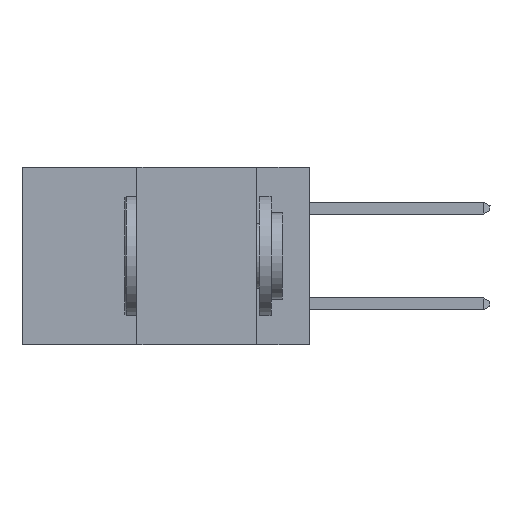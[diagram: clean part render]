
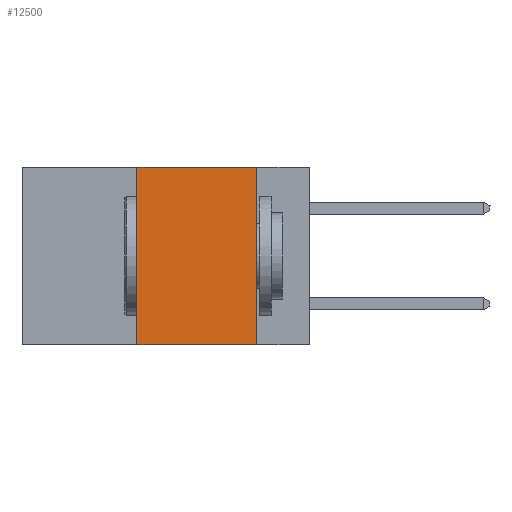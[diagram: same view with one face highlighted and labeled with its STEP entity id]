
A CAD part, left-side view. The second image highlights one B-rep face of the part: STEP entity #12500.
In plain terms, the highlighted planar face has unit normal (-1, 0, 0).
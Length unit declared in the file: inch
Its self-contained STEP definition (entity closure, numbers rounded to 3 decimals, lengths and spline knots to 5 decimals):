
#22 = ORIENTED_EDGE ( 'NONE', *, *, #7633, .F. ) ;
#242 = ORIENTED_EDGE ( 'NONE', *, *, #12107, .F. ) ;
#319 = ORIENTED_EDGE ( 'NONE', *, *, #15485, .F. ) ;
#1530 = ORIENTED_EDGE ( 'NONE', *, *, #19154, .T. ) ;
#2858 = VERTEX_POINT ( 'NONE', #14067 ) ;
#2990 = CARTESIAN_POINT ( 'NONE',  ( 0., 0.11, 0. ) ) ;
#3079 = VECTOR ( 'NONE', #8066, 39.37008 ) ;
#3579 = LINE ( 'NONE', #18610, #3079 ) ;
#5143 = VERTEX_POINT ( 'NONE', #9346 ) ;
#5203 = CARTESIAN_POINT ( 'NONE',  ( 0., 0.11, -0.37 ) ) ;
#5963 = AXIS2_PLACEMENT_3D ( 'NONE', #9404, #16978, #7877 ) ;
#6797 = CARTESIAN_POINT ( 'NONE',  ( 0., 0.6, 0. ) ) ;
#7076 = VERTEX_POINT ( 'NONE', #5203 ) ;
#7633 = EDGE_CURVE ( 'NONE', #13668, #7076, #3579, .T. ) ;
#7877 = DIRECTION ( 'NONE',  ( 0., 0., -1. ) ) ;
#8066 = DIRECTION ( 'NONE',  ( 0., 0., -1. ) ) ;
#9346 = CARTESIAN_POINT ( 'NONE',  ( 0., 0.36, -0.37 ) ) ;
#9404 = CARTESIAN_POINT ( 'NONE',  ( 0., 0.6, 0. ) ) ;
#9689 = CARTESIAN_POINT ( 'NONE',  ( 0., 0.36, 0. ) ) ;
#10066 = LINE ( 'NONE', #9689, #17588 ) ;
#10252 = EDGE_LOOP ( 'NONE', ( #22, #242, #319, #1530 ) ) ;
#10405 = CARTESIAN_POINT ( 'NONE',  ( 0., 0.6, -0.37 ) ) ;
#11948 = FACE_OUTER_BOUND ( 'NONE', #10252, .T. ) ;
#11968 = LINE ( 'NONE', #6797, #15439 ) ;
#12107 = EDGE_CURVE ( 'NONE', #2858, #13668, #11968, .T. ) ;
#12474 = PLANE ( 'NONE',  #5963 ) ;
#12500 = ADVANCED_FACE ( 'NONE', ( #11948 ), #12474, .F. ) ;
#13668 = VERTEX_POINT ( 'NONE', #2990 ) ;
#14067 = CARTESIAN_POINT ( 'NONE',  ( 0., 0.36, 0. ) ) ;
#15439 = VECTOR ( 'NONE', #18910, 39.37008 ) ;
#15485 = EDGE_CURVE ( 'NONE', #5143, #2858, #10066, .T. ) ;
#15713 = DIRECTION ( 'NONE',  ( 0., 0., 1. ) ) ;
#16945 = VECTOR ( 'NONE', #19332, 39.37008 ) ;
#16978 = DIRECTION ( 'NONE',  ( 1., 0., 0. ) ) ;
#17588 = VECTOR ( 'NONE', #15713, 39.37008 ) ;
#18610 = CARTESIAN_POINT ( 'NONE',  ( 0., 0.11, 0. ) ) ;
#18910 = DIRECTION ( 'NONE',  ( 0., -1., 0. ) ) ;
#19154 = EDGE_CURVE ( 'NONE', #5143, #7076, #19462, .T. ) ;
#19332 = DIRECTION ( 'NONE',  ( 0., -1., 0. ) ) ;
#19462 = LINE ( 'NONE', #10405, #16945 ) ;
